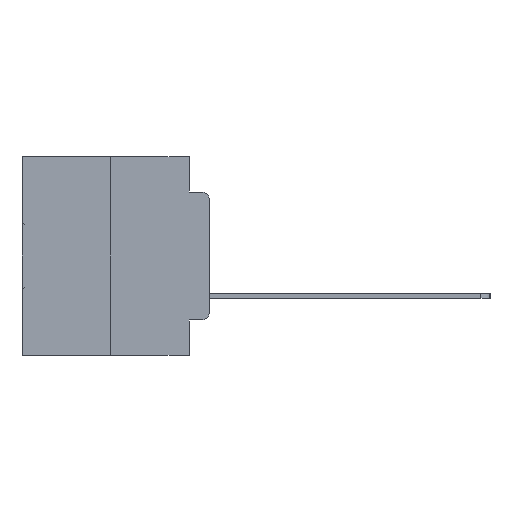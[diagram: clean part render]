
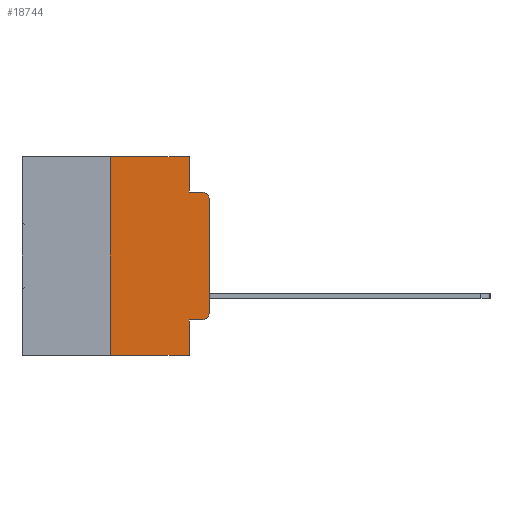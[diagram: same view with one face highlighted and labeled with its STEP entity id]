
A CAD part, left-side view. The second image highlights one B-rep face of the part: STEP entity #18744.
In plain terms, the highlighted planar face has unit normal (-1, 0, 0).
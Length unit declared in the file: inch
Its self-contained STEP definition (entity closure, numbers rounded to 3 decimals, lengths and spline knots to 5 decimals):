
#27 = VERTEX_POINT ( 'NONE', #12399 ) ;
#1023 = DIRECTION ( 'NONE',  ( 0., -1., 0. ) ) ;
#2171 = VECTOR ( 'NONE', #30752, 39.37008 ) ;
#2517 = ORIENTED_EDGE ( 'NONE', *, *, #19470, .F. ) ;
#3364 = LINE ( 'NONE', #13380, #17420 ) ;
#3445 = DIRECTION ( 'NONE',  ( 0., 0., -1. ) ) ;
#3559 = VERTEX_POINT ( 'NONE', #23934 ) ;
#3749 = ORIENTED_EDGE ( 'NONE', *, *, #14273, .F. ) ;
#5723 = CARTESIAN_POINT ( 'NONE',  ( 0., 0.25, -0.5 ) ) ;
#5919 = CIRCLE ( 'NONE', #12809, 0.02 ) ;
#6068 = LINE ( 'NONE', #7382, #20045 ) ;
#7382 = CARTESIAN_POINT ( 'NONE',  ( 0., 0., 0. ) ) ;
#7605 = AXIS2_PLACEMENT_3D ( 'NONE', #26016, #10459, #28589 ) ;
#7710 = VECTOR ( 'NONE', #18221, 39.37008 ) ;
#7771 = PLANE ( 'NONE',  #7605 ) ;
#8398 = ORIENTED_EDGE ( 'NONE', *, *, #8965, .T. ) ;
#8892 = LINE ( 'NONE', #32440, #21980 ) ;
#8965 = EDGE_CURVE ( 'NONE', #23610, #26024, #5919, .T. ) ;
#9195 = ORIENTED_EDGE ( 'NONE', *, *, #14726, .T. ) ;
#10459 = DIRECTION ( 'NONE',  ( 1., 0., 0. ) ) ;
#10827 = ORIENTED_EDGE ( 'NONE', *, *, #17727, .F. ) ;
#11026 = FACE_OUTER_BOUND ( 'NONE', #25804, .T. ) ;
#12399 = CARTESIAN_POINT ( 'NONE',  ( 0., 0.051, -0.0885 ) ) ;
#12527 = EDGE_CURVE ( 'NONE', #3559, #23610, #23215, .T. ) ;
#12809 = AXIS2_PLACEMENT_3D ( 'NONE', #28405, #12903, #31014 ) ;
#12903 = DIRECTION ( 'NONE',  ( -1., 0., 0. ) ) ;
#13275 = VERTEX_POINT ( 'NONE', #23725 ) ;
#13380 = CARTESIAN_POINT ( 'NONE',  ( 0., 0.473, 0. ) ) ;
#13439 = AXIS2_PLACEMENT_3D ( 'NONE', #31441, #15985, #3445 ) ;
#14273 = EDGE_CURVE ( 'NONE', #3559, #32883, #23534, .T. ) ;
#14726 = EDGE_CURVE ( 'NONE', #15648, #32883, #30010, .T. ) ;
#14746 = LINE ( 'NONE', #31108, #7710 ) ;
#15648 = VERTEX_POINT ( 'NONE', #5723 ) ;
#15824 = VECTOR ( 'NONE', #26758, 39.37008 ) ;
#15985 = DIRECTION ( 'NONE',  ( -1., 0., 0. ) ) ;
#16026 = EDGE_CURVE ( 'NONE', #15648, #18608, #33518, .T. ) ;
#16065 = CARTESIAN_POINT ( 'NONE',  ( 0., 0.051, -0.5 ) ) ;
#16476 = CARTESIAN_POINT ( 'NONE',  ( 0., 0.051, 0. ) ) ;
#17420 = VECTOR ( 'NONE', #31486, 39.37008 ) ;
#17727 = EDGE_CURVE ( 'NONE', #26003, #27, #14746, .T. ) ;
#18221 = DIRECTION ( 'NONE',  ( 0., 0., -1. ) ) ;
#18608 = VERTEX_POINT ( 'NONE', #22803 ) ;
#18744 = ADVANCED_FACE ( 'NONE', ( #11026 ), #7771, .F. ) ;
#19470 = EDGE_CURVE ( 'NONE', #27, #22274, #8892, .T. ) ;
#20045 = VECTOR ( 'NONE', #25655, 39.37008 ) ;
#20525 = CARTESIAN_POINT ( 'NONE',  ( 0., 0.25, 0. ) ) ;
#21231 = EDGE_CURVE ( 'NONE', #13275, #22274, #29391, .T. ) ;
#21980 = VECTOR ( 'NONE', #1023, 39.37008 ) ;
#22274 = VERTEX_POINT ( 'NONE', #22619 ) ;
#22619 = CARTESIAN_POINT ( 'NONE',  ( 0., 0.02, -0.0885 ) ) ;
#22803 = CARTESIAN_POINT ( 'NONE',  ( 0., 0.25, 0. ) ) ;
#23178 = VECTOR ( 'NONE', #28618, 39.37008 ) ;
#23215 = LINE ( 'NONE', #28140, #2171 ) ;
#23520 = ORIENTED_EDGE ( 'NONE', *, *, #12527, .T. ) ;
#23534 = LINE ( 'NONE', #16476, #15824 ) ;
#23610 = VERTEX_POINT ( 'NONE', #26153 ) ;
#23725 = CARTESIAN_POINT ( 'NONE',  ( 0., 0., -0.1085 ) ) ;
#23934 = CARTESIAN_POINT ( 'NONE',  ( 0., 0.051, -0.4115 ) ) ;
#24695 = EDGE_CURVE ( 'NONE', #26024, #13275, #6068, .T. ) ;
#25655 = DIRECTION ( 'NONE',  ( 0., 0., 1. ) ) ;
#25804 = EDGE_LOOP ( 'NONE', ( #27523, #33998, #2517, #10827, #27072, #33573, #9195, #3749, #23520, #8398 ) ) ;
#26003 = VERTEX_POINT ( 'NONE', #28823 ) ;
#26016 = CARTESIAN_POINT ( 'NONE',  ( 0., 0.473, 0. ) ) ;
#26024 = VERTEX_POINT ( 'NONE', #31678 ) ;
#26153 = CARTESIAN_POINT ( 'NONE',  ( 0., 0.02, -0.4115 ) ) ;
#26758 = DIRECTION ( 'NONE',  ( 0., 0., -1. ) ) ;
#27072 = ORIENTED_EDGE ( 'NONE', *, *, #27294, .F. ) ;
#27294 = EDGE_CURVE ( 'NONE', #18608, #26003, #3364, .T. ) ;
#27523 = ORIENTED_EDGE ( 'NONE', *, *, #24695, .T. ) ;
#28140 = CARTESIAN_POINT ( 'NONE',  ( 0., 0.051, -0.4115 ) ) ;
#28292 = DIRECTION ( 'NONE',  ( 0., 0., 1. ) ) ;
#28405 = CARTESIAN_POINT ( 'NONE',  ( 0., 0.02, -0.3915 ) ) ;
#28589 = DIRECTION ( 'NONE',  ( 0., 0., -1. ) ) ;
#28618 = DIRECTION ( 'NONE',  ( 0., -1., 0. ) ) ;
#28823 = CARTESIAN_POINT ( 'NONE',  ( 0., 0.051, 0. ) ) ;
#29391 = CIRCLE ( 'NONE', #13439, 0.02 ) ;
#30010 = LINE ( 'NONE', #31120, #23178 ) ;
#30752 = DIRECTION ( 'NONE',  ( 0., -1., 0. ) ) ;
#31014 = DIRECTION ( 'NONE',  ( 0., 0., -1. ) ) ;
#31108 = CARTESIAN_POINT ( 'NONE',  ( 0., 0.051, 0. ) ) ;
#31120 = CARTESIAN_POINT ( 'NONE',  ( 0., 0.473, -0.5 ) ) ;
#31441 = CARTESIAN_POINT ( 'NONE',  ( 0., 0.02, -0.1085 ) ) ;
#31486 = DIRECTION ( 'NONE',  ( 0., -1., 0. ) ) ;
#31678 = CARTESIAN_POINT ( 'NONE',  ( 0., 0., -0.3915 ) ) ;
#32440 = CARTESIAN_POINT ( 'NONE',  ( 0., 0.051, -0.0885 ) ) ;
#32722 = VECTOR ( 'NONE', #28292, 39.37008 ) ;
#32883 = VERTEX_POINT ( 'NONE', #16065 ) ;
#33518 = LINE ( 'NONE', #20525, #32722 ) ;
#33573 = ORIENTED_EDGE ( 'NONE', *, *, #16026, .F. ) ;
#33998 = ORIENTED_EDGE ( 'NONE', *, *, #21231, .T. ) ;
